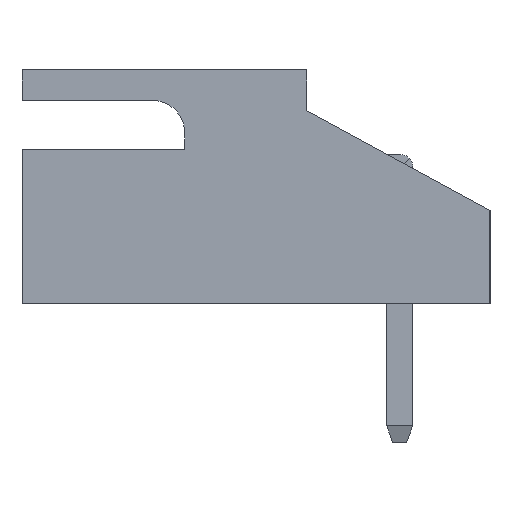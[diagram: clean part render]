
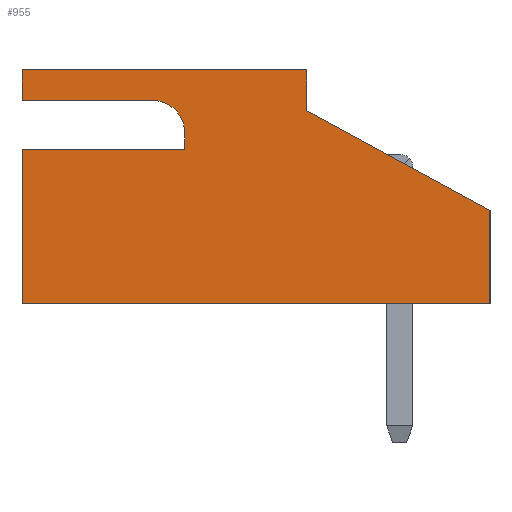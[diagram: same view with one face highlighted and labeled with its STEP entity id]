
A CAD part, left-side view. The second image highlights one B-rep face of the part: STEP entity #955.
In plain terms, the highlighted planar face has unit normal (-1, 0, 0).
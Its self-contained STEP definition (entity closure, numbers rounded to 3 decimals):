
#264 = VECTOR ( 'NONE', #3719, 1000. ) ;
#297 = LINE ( 'NONE', #1718, #587 ) ;
#337 = ORIENTED_EDGE ( 'NONE', *, *, #2323, .T. ) ;
#339 = VERTEX_POINT ( 'NONE', #700 ) ;
#423 = VERTEX_POINT ( 'NONE', #6000 ) ;
#587 = VECTOR ( 'NONE', #3812, 1000. ) ;
#654 = VERTEX_POINT ( 'NONE', #4431 ) ;
#700 = CARTESIAN_POINT ( 'NONE',  ( -15., 7., 2.875 ) ) ;
#742 = VERTEX_POINT ( 'NONE', #5627 ) ;
#910 = LINE ( 'NONE', #2895, #2335 ) ;
#919 = DIRECTION ( 'NONE',  ( 0., -0.878, -0.478 ) ) ;
#955 = ADVANCED_FACE ( 'NONE', ( #6186 ), #1792, .F. ) ;
#1000 = CARTESIAN_POINT ( 'NONE',  ( -15., 7., 2.125 ) ) ;
#1171 = LINE ( 'NONE', #6214, #4756 ) ;
#1272 = CARTESIAN_POINT ( 'NONE',  ( -15., 7., -2.875 ) ) ;
#1359 = EDGE_CURVE ( 'NONE', #339, #1415, #1171, .T. ) ;
#1374 = EDGE_CURVE ( 'NONE', #4967, #3209, #3188, .T. ) ;
#1415 = VERTEX_POINT ( 'NONE', #4137 ) ;
#1460 = EDGE_CURVE ( 'NONE', #5754, #654, #3960, .T. ) ;
#1469 = CARTESIAN_POINT ( 'NONE',  ( -15., 7., -2.875 ) ) ;
#1515 = VECTOR ( 'NONE', #4005, 1000. ) ;
#1524 = LINE ( 'NONE', #4102, #1515 ) ;
#1616 = EDGE_LOOP ( 'NONE', ( #3056, #5716, #2470, #6415, #3177, #3138, #337, #4931, #5674, #4999, #5743 ) ) ;
#1718 = CARTESIAN_POINT ( 'NONE',  ( -15., -4.5, -0.575 ) ) ;
#1792 = PLANE ( 'NONE',  #4239 ) ;
#1846 = DIRECTION ( 'NONE',  ( 0., 0., -1. ) ) ;
#1917 = VECTOR ( 'NONE', #1846, 1000. ) ;
#2179 = DIRECTION ( 'NONE',  ( 0., -1., 0. ) ) ;
#2243 = VECTOR ( 'NONE', #5250, 1000. ) ;
#2323 = EDGE_CURVE ( 'NONE', #4967, #6025, #3729, .T. ) ;
#2335 = VECTOR ( 'NONE', #4060, 1000. ) ;
#2359 = VECTOR ( 'NONE', #919, 1000. ) ;
#2470 = ORIENTED_EDGE ( 'NONE', *, *, #5219, .T. ) ;
#2692 = CARTESIAN_POINT ( 'NONE',  ( -15., 7., -2.875 ) ) ;
#2895 = CARTESIAN_POINT ( 'NONE',  ( -15., 0., -2.875 ) ) ;
#3042 = EDGE_CURVE ( 'NONE', #5754, #339, #1524, .T. ) ;
#3056 = ORIENTED_EDGE ( 'NONE', *, *, #3042, .F. ) ;
#3111 = CARTESIAN_POINT ( 'NONE',  ( -15., 7., 2.125 ) ) ;
#3138 = ORIENTED_EDGE ( 'NONE', *, *, #1374, .F. ) ;
#3177 = ORIENTED_EDGE ( 'NONE', *, *, #5213, .T. ) ;
#3188 = LINE ( 'NONE', #1272, #5485 ) ;
#3193 = CARTESIAN_POINT ( 'NONE',  ( -15., 7., -2.875 ) ) ;
#3209 = VERTEX_POINT ( 'NONE', #3283 ) ;
#3244 = DIRECTION ( 'NONE',  ( 0., 0., 1. ) ) ;
#3250 = EDGE_CURVE ( 'NONE', #742, #6025, #297, .T. ) ;
#3283 = CARTESIAN_POINT ( 'NONE',  ( -15., 7., 0.925 ) ) ;
#3311 = CARTESIAN_POINT ( 'NONE',  ( -15., 3., 0.925 ) ) ;
#3359 = CARTESIAN_POINT ( 'NONE',  ( -15., 3., 1.325 ) ) ;
#3459 = DIRECTION ( 'NONE',  ( 0., -1., 0. ) ) ;
#3516 = CARTESIAN_POINT ( 'NONE',  ( -15., -4.5, -2.875 ) ) ;
#3641 = EDGE_CURVE ( 'NONE', #4812, #742, #5419, .T. ) ;
#3719 = DIRECTION ( 'NONE',  ( 0., 1., 0. ) ) ;
#3729 = LINE ( 'NONE', #2692, #2243 ) ;
#3746 = DIRECTION ( 'NONE',  ( 1., 0., 0. ) ) ;
#3776 = DIRECTION ( 'NONE',  ( 1., 0., 0. ) ) ;
#3812 = DIRECTION ( 'NONE',  ( 0., 0., -1. ) ) ;
#3960 = LINE ( 'NONE', #1000, #4868 ) ;
#4005 = DIRECTION ( 'NONE',  ( 0., 0., 1. ) ) ;
#4060 = DIRECTION ( 'NONE',  ( 0., 0., 1. ) ) ;
#4102 = CARTESIAN_POINT ( 'NONE',  ( -15., 7., -2.875 ) ) ;
#4114 = CIRCLE ( 'NONE', #6388, 0.8 ) ;
#4137 = CARTESIAN_POINT ( 'NONE',  ( -15., 0., 2.875 ) ) ;
#4239 = AXIS2_PLACEMENT_3D ( 'NONE', #3193, #3776, #4715 ) ;
#4354 = CARTESIAN_POINT ( 'NONE',  ( -15., 0., 1.875 ) ) ;
#4422 = VERTEX_POINT ( 'NONE', #3311 ) ;
#4431 = CARTESIAN_POINT ( 'NONE',  ( -15., 3.8, 2.125 ) ) ;
#4715 = DIRECTION ( 'NONE',  ( 0., 0., -1. ) ) ;
#4720 = EDGE_CURVE ( 'NONE', #423, #4422, #4830, .T. ) ;
#4756 = VECTOR ( 'NONE', #2179, 1000. ) ;
#4812 = VERTEX_POINT ( 'NONE', #4354 ) ;
#4830 = LINE ( 'NONE', #3359, #1917 ) ;
#4868 = VECTOR ( 'NONE', #3459, 1000. ) ;
#4931 = ORIENTED_EDGE ( 'NONE', *, *, #3250, .F. ) ;
#4967 = VERTEX_POINT ( 'NONE', #1469 ) ;
#4999 = ORIENTED_EDGE ( 'NONE', *, *, #5742, .T. ) ;
#5204 = LINE ( 'NONE', #6405, #264 ) ;
#5213 = EDGE_CURVE ( 'NONE', #4422, #3209, #5204, .T. ) ;
#5219 = EDGE_CURVE ( 'NONE', #654, #423, #4114, .T. ) ;
#5250 = DIRECTION ( 'NONE',  ( 0., -1., 0. ) ) ;
#5419 = LINE ( 'NONE', #5847, #2359 ) ;
#5485 = VECTOR ( 'NONE', #3244, 1000. ) ;
#5627 = CARTESIAN_POINT ( 'NONE',  ( -15., -4.5, -0.575 ) ) ;
#5674 = ORIENTED_EDGE ( 'NONE', *, *, #3641, .F. ) ;
#5699 = CARTESIAN_POINT ( 'NONE',  ( -15., 3.8, 1.325 ) ) ;
#5716 = ORIENTED_EDGE ( 'NONE', *, *, #1460, .T. ) ;
#5742 = EDGE_CURVE ( 'NONE', #4812, #1415, #910, .T. ) ;
#5743 = ORIENTED_EDGE ( 'NONE', *, *, #1359, .F. ) ;
#5754 = VERTEX_POINT ( 'NONE', #3111 ) ;
#5847 = CARTESIAN_POINT ( 'NONE',  ( -15., 0., 1.875 ) ) ;
#6000 = CARTESIAN_POINT ( 'NONE',  ( -15., 3., 1.325 ) ) ;
#6025 = VERTEX_POINT ( 'NONE', #3516 ) ;
#6186 = FACE_OUTER_BOUND ( 'NONE', #1616, .T. ) ;
#6214 = CARTESIAN_POINT ( 'NONE',  ( -15., 7., 2.875 ) ) ;
#6288 = DIRECTION ( 'NONE',  ( 0., 0., -1. ) ) ;
#6388 = AXIS2_PLACEMENT_3D ( 'NONE', #5699, #3746, #6288 ) ;
#6405 = CARTESIAN_POINT ( 'NONE',  ( -15., 7., 0.925 ) ) ;
#6415 = ORIENTED_EDGE ( 'NONE', *, *, #4720, .T. ) ;
